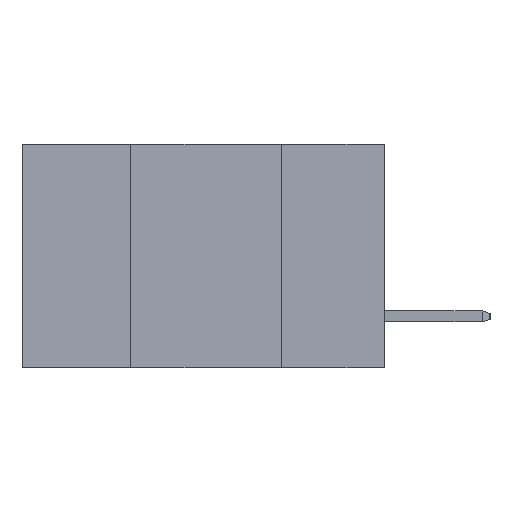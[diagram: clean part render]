
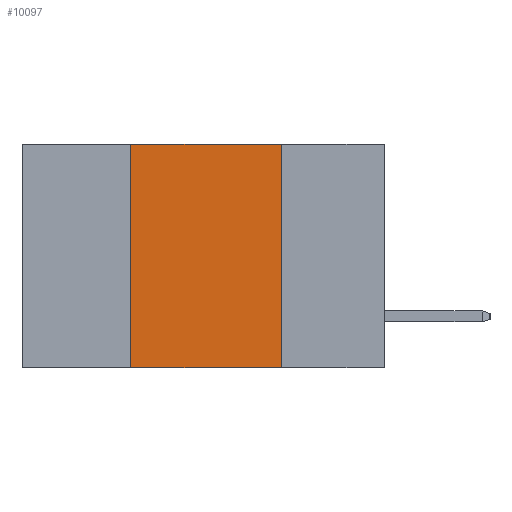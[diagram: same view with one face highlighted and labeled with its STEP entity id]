
A CAD part, left-side view. The second image highlights one B-rep face of the part: STEP entity #10097.
In plain terms, the highlighted planar face has unit normal (-1, 0, 0).
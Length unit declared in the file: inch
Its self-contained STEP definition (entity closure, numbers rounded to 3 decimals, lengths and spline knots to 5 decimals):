
#171 = LINE ( 'NONE', #366, #16371 ) ;
#289 = VECTOR ( 'NONE', #11401, 39.37008 ) ;
#366 = CARTESIAN_POINT ( 'NONE',  ( 0., 0.42, 0. ) ) ;
#446 = DIRECTION ( 'NONE',  ( 0., 0., -1. ) ) ;
#1086 = EDGE_CURVE ( 'NONE', #16459, #9235, #4412, .T. ) ;
#2157 = EDGE_CURVE ( 'NONE', #15203, #9235, #11997, .T. ) ;
#2339 = FACE_OUTER_BOUND ( 'NONE', #11954, .T. ) ;
#2712 = CARTESIAN_POINT ( 'NONE',  ( 0., 0.6, 0. ) ) ;
#4246 = ORIENTED_EDGE ( 'NONE', *, *, #9979, .F. ) ;
#4412 = LINE ( 'NONE', #11032, #289 ) ;
#5093 = ORIENTED_EDGE ( 'NONE', *, *, #2157, .T. ) ;
#6670 = CARTESIAN_POINT ( 'NONE',  ( 0., 0.6, 0. ) ) ;
#7344 = VECTOR ( 'NONE', #12578, 39.37008 ) ;
#9235 = VERTEX_POINT ( 'NONE', #15886 ) ;
#9726 = DIRECTION ( 'NONE',  ( 0., 0., 1. ) ) ;
#9809 = DIRECTION ( 'NONE',  ( 1., 0., 0. ) ) ;
#9979 = EDGE_CURVE ( 'NONE', #15203, #16402, #171, .T. ) ;
#10097 = ADVANCED_FACE ( 'NONE', ( #2339 ), #19262, .F. ) ;
#11032 = CARTESIAN_POINT ( 'NONE',  ( 0., 0.17, 0. ) ) ;
#11217 = AXIS2_PLACEMENT_3D ( 'NONE', #6670, #9809, #446 ) ;
#11401 = DIRECTION ( 'NONE',  ( 0., 0., -1. ) ) ;
#11954 = EDGE_LOOP ( 'NONE', ( #20057, #13219, #4246, #5093 ) ) ;
#11997 = LINE ( 'NONE', #19188, #7344 ) ;
#12084 = VECTOR ( 'NONE', #15282, 39.37008 ) ;
#12578 = DIRECTION ( 'NONE',  ( 0., -1., 0. ) ) ;
#13219 = ORIENTED_EDGE ( 'NONE', *, *, #16307, .F. ) ;
#15203 = VERTEX_POINT ( 'NONE', #18783 ) ;
#15282 = DIRECTION ( 'NONE',  ( 0., -1., 0. ) ) ;
#15422 = CARTESIAN_POINT ( 'NONE',  ( 0., 0.42, 0. ) ) ;
#15772 = LINE ( 'NONE', #2712, #12084 ) ;
#15886 = CARTESIAN_POINT ( 'NONE',  ( 0., 0.17, -0.37 ) ) ;
#16307 = EDGE_CURVE ( 'NONE', #16402, #16459, #15772, .T. ) ;
#16371 = VECTOR ( 'NONE', #9726, 39.37008 ) ;
#16402 = VERTEX_POINT ( 'NONE', #15422 ) ;
#16459 = VERTEX_POINT ( 'NONE', #18813 ) ;
#18783 = CARTESIAN_POINT ( 'NONE',  ( 0., 0.42, -0.37 ) ) ;
#18813 = CARTESIAN_POINT ( 'NONE',  ( 0., 0.17, 0. ) ) ;
#19188 = CARTESIAN_POINT ( 'NONE',  ( 0., 0.6, -0.37 ) ) ;
#19262 = PLANE ( 'NONE',  #11217 ) ;
#20057 = ORIENTED_EDGE ( 'NONE', *, *, #1086, .F. ) ;
